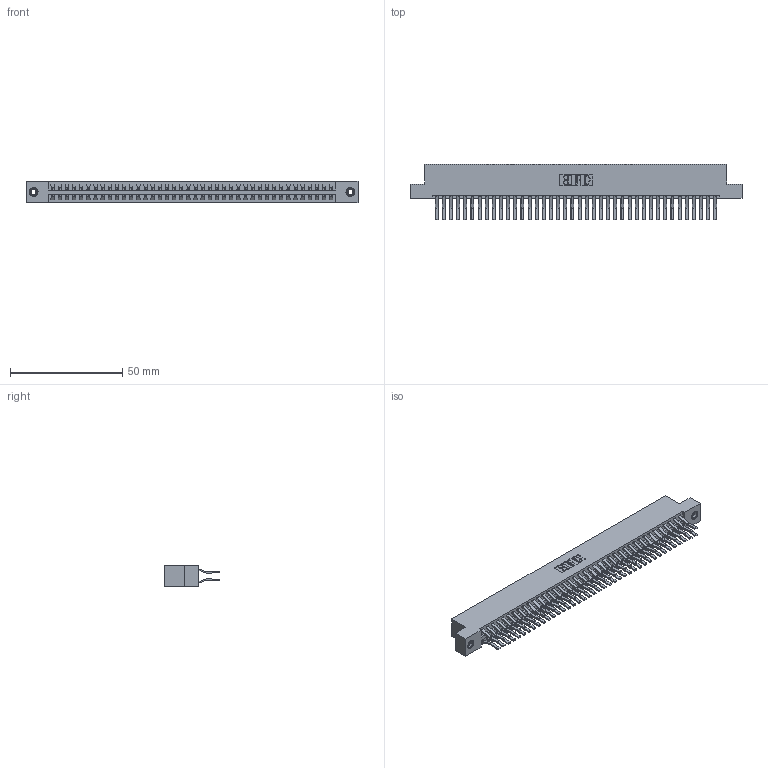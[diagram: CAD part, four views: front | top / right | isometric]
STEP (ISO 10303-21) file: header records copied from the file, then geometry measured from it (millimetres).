
FILE_DESCRIPTION (( 'STEP AP203' ), '1' );
FILE_NAME ('396-080-560-208.STEP', '2019-10-30T23:09:48', ( '' ), ( '' ), 'SwSTEP 2.0', 'SolidWorks 2016', '' );
FILE_SCHEMA (( 'CONFIG_CONTROL_DESIGN' ));
Length unit declared in the file: inch
Products named in the file (4): 345-292-001_560 Tail; 396-080-560-208; 346 Part_Flush Mounting Lugs - 0.156 Dia-TI; 345-250-001_345-250-003-102
Assembly tree (83 placements, depth 2):
  396-080-560-208
    346 Part_Flush Mounting Lugs - 0.156 Dia-TI
    345-292-001_560 Tail  x80
    345-250-001_345-250-003-102  x2
Bounding box: 147.57 x 24.78 x 9.4 mm (x, y, z)
Volume: 14892.6 mm3; surface area: 21858.5 mm2
Topology: 83 solids, 83 shells, 4502 faces, 13345 edges, 8782 vertices
Faces by surface type: plane 2908, cylinder 1578, cone 12, torus 4
Entity records: 27648 total; most frequent: CARTESIAN_POINT 4543, ORIENTED_EDGE 4470, DIRECTION 4085, EDGE_CURVE 2235, VECTOR 1919, LINE 1919, VERTEX_POINT 1484, AXIS2_PLACEMENT_3D 1083
